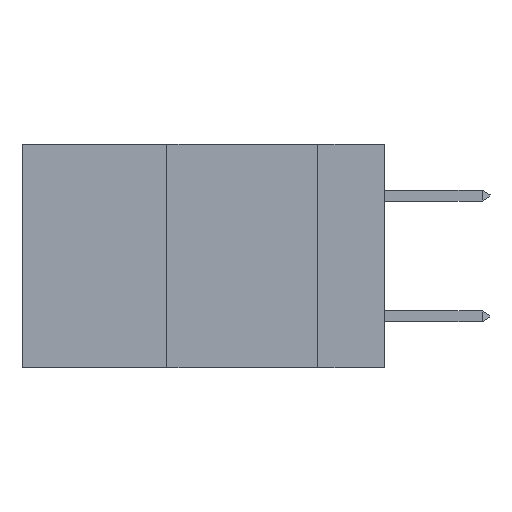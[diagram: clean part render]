
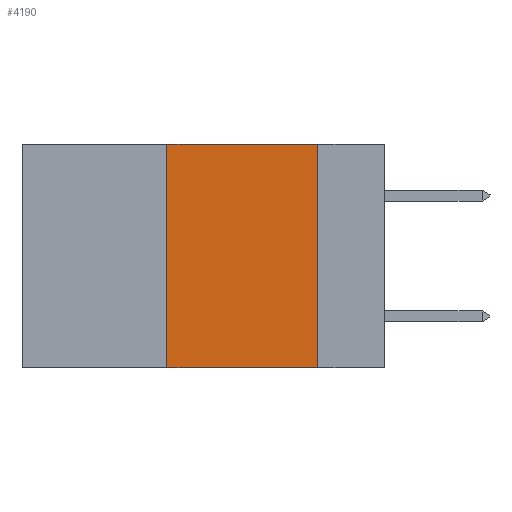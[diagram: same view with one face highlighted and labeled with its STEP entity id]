
A CAD part, left-side view. The second image highlights one B-rep face of the part: STEP entity #4190.
In plain terms, the highlighted planar face has unit normal (-1, 0, 0).
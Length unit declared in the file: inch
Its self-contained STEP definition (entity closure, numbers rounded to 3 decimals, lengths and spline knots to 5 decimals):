
#289 = VERTEX_POINT ( 'NONE', #20103 ) ;
#1336 = CARTESIAN_POINT ( 'NONE',  ( 0., 0.11, 0. ) ) ;
#2423 = CARTESIAN_POINT ( 'NONE',  ( 0., 0.36, 0. ) ) ;
#2713 = DIRECTION ( 'NONE',  ( 0., 0., -1. ) ) ;
#2811 = PLANE ( 'NONE',  #15841 ) ;
#2945 = VECTOR ( 'NONE', #29789, 39.37008 ) ;
#3008 = DIRECTION ( 'NONE',  ( 1., 0., 0. ) ) ;
#3868 = EDGE_CURVE ( 'NONE', #289, #27250, #5690, .T. ) ;
#4059 = DIRECTION ( 'NONE',  ( 0., 0., -1. ) ) ;
#4190 = ADVANCED_FACE ( 'NONE', ( #7136 ), #2811, .F. ) ;
#5690 = LINE ( 'NONE', #2423, #28058 ) ;
#5898 = VERTEX_POINT ( 'NONE', #21077 ) ;
#6285 = EDGE_CURVE ( 'NONE', #27250, #25702, #21400, .T. ) ;
#6291 = EDGE_LOOP ( 'NONE', ( #28666, #29764, #18863, #24604 ) ) ;
#7136 = FACE_OUTER_BOUND ( 'NONE', #6291, .T. ) ;
#7796 = EDGE_CURVE ( 'NONE', #289, #5898, #11617, .T. ) ;
#8975 = EDGE_CURVE ( 'NONE', #25702, #5898, #27366, .T. ) ;
#9640 = CARTESIAN_POINT ( 'NONE',  ( 0., 0.6, -0.37 ) ) ;
#10030 = CARTESIAN_POINT ( 'NONE',  ( 0., 0.6, 0. ) ) ;
#11617 = LINE ( 'NONE', #9640, #18469 ) ;
#14007 = CARTESIAN_POINT ( 'NONE',  ( 0., 0.11, 0. ) ) ;
#14394 = DIRECTION ( 'NONE',  ( 0., 0., 1. ) ) ;
#15841 = AXIS2_PLACEMENT_3D ( 'NONE', #10030, #3008, #2713 ) ;
#18469 = VECTOR ( 'NONE', #28021, 39.37008 ) ;
#18863 = ORIENTED_EDGE ( 'NONE', *, *, #3868, .F. ) ;
#20103 = CARTESIAN_POINT ( 'NONE',  ( 0., 0.36, -0.37 ) ) ;
#21077 = CARTESIAN_POINT ( 'NONE',  ( 0., 0.11, -0.37 ) ) ;
#21400 = LINE ( 'NONE', #24949, #2945 ) ;
#23505 = CARTESIAN_POINT ( 'NONE',  ( 0., 0.36, 0. ) ) ;
#24604 = ORIENTED_EDGE ( 'NONE', *, *, #7796, .T. ) ;
#24949 = CARTESIAN_POINT ( 'NONE',  ( 0., 0.6, 0. ) ) ;
#25702 = VERTEX_POINT ( 'NONE', #14007 ) ;
#26603 = VECTOR ( 'NONE', #4059, 39.37008 ) ;
#27250 = VERTEX_POINT ( 'NONE', #23505 ) ;
#27366 = LINE ( 'NONE', #1336, #26603 ) ;
#28021 = DIRECTION ( 'NONE',  ( 0., -1., 0. ) ) ;
#28058 = VECTOR ( 'NONE', #14394, 39.37008 ) ;
#28666 = ORIENTED_EDGE ( 'NONE', *, *, #8975, .F. ) ;
#29764 = ORIENTED_EDGE ( 'NONE', *, *, #6285, .F. ) ;
#29789 = DIRECTION ( 'NONE',  ( 0., -1., 0. ) ) ;
